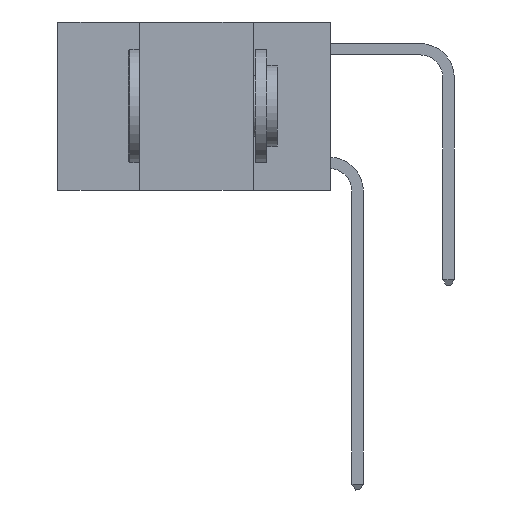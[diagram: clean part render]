
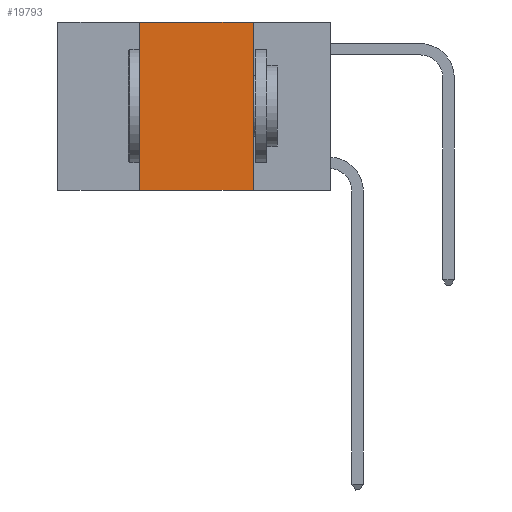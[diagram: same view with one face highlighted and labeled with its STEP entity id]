
A CAD part, left-side view. The second image highlights one B-rep face of the part: STEP entity #19793.
In plain terms, the highlighted planar face has unit normal (-1, 0, 0).
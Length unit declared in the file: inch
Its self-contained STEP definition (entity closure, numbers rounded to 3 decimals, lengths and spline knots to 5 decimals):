
#1401 = CARTESIAN_POINT ( 'NONE',  ( 0., 0.42, -0.37 ) ) ;
#1426 = CARTESIAN_POINT ( 'NONE',  ( 0., 0.42, 0. ) ) ;
#1577 = CARTESIAN_POINT ( 'NONE',  ( 0., 0.42, 0. ) ) ;
#2599 = EDGE_CURVE ( 'NONE', #12961, #17597, #9958, .T. ) ;
#8161 = EDGE_LOOP ( 'NONE', ( #20358, #10161, #29308, #23967 ) ) ;
#8846 = PLANE ( 'NONE',  #21589 ) ;
#9958 = LINE ( 'NONE', #28740, #21608 ) ;
#10161 = ORIENTED_EDGE ( 'NONE', *, *, #21320, .F. ) ;
#12317 = FACE_OUTER_BOUND ( 'NONE', #8161, .T. ) ;
#12961 = VERTEX_POINT ( 'NONE', #29725 ) ;
#13458 = DIRECTION ( 'NONE',  ( 0., 0., -1. ) ) ;
#14220 = CARTESIAN_POINT ( 'NONE',  ( 0., 0.6, -0.37 ) ) ;
#17033 = EDGE_CURVE ( 'NONE', #17584, #22737, #29746, .T. ) ;
#17355 = DIRECTION ( 'NONE',  ( 0., 0., -1. ) ) ;
#17584 = VERTEX_POINT ( 'NONE', #1401 ) ;
#17597 = VERTEX_POINT ( 'NONE', #24671 ) ;
#17839 = LINE ( 'NONE', #14220, #23286 ) ;
#18950 = DIRECTION ( 'NONE',  ( 0., -1., 0. ) ) ;
#19380 = EDGE_CURVE ( 'NONE', #17584, #17597, #17839, .T. ) ;
#19793 = ADVANCED_FACE ( 'NONE', ( #12317 ), #8846, .F. ) ;
#20276 = LINE ( 'NONE', #24219, #25678 ) ;
#20358 = ORIENTED_EDGE ( 'NONE', *, *, #2599, .F. ) ;
#21320 = EDGE_CURVE ( 'NONE', #22737, #12961, #20276, .T. ) ;
#21589 = AXIS2_PLACEMENT_3D ( 'NONE', #25064, #27364, #13458 ) ;
#21608 = VECTOR ( 'NONE', #17355, 39.37008 ) ;
#21900 = DIRECTION ( 'NONE',  ( 0., -1., 0. ) ) ;
#22261 = DIRECTION ( 'NONE',  ( 0., 0., 1. ) ) ;
#22737 = VERTEX_POINT ( 'NONE', #1577 ) ;
#23286 = VECTOR ( 'NONE', #18950, 39.37008 ) ;
#23687 = VECTOR ( 'NONE', #22261, 39.37008 ) ;
#23967 = ORIENTED_EDGE ( 'NONE', *, *, #19380, .T. ) ;
#24219 = CARTESIAN_POINT ( 'NONE',  ( 0., 0.6, 0. ) ) ;
#24671 = CARTESIAN_POINT ( 'NONE',  ( 0., 0.17, -0.37 ) ) ;
#25064 = CARTESIAN_POINT ( 'NONE',  ( 0., 0.6, 0. ) ) ;
#25678 = VECTOR ( 'NONE', #21900, 39.37008 ) ;
#27364 = DIRECTION ( 'NONE',  ( 1., 0., 0. ) ) ;
#28740 = CARTESIAN_POINT ( 'NONE',  ( 0., 0.17, 0. ) ) ;
#29308 = ORIENTED_EDGE ( 'NONE', *, *, #17033, .F. ) ;
#29725 = CARTESIAN_POINT ( 'NONE',  ( 0., 0.17, 0. ) ) ;
#29746 = LINE ( 'NONE', #1426, #23687 ) ;
